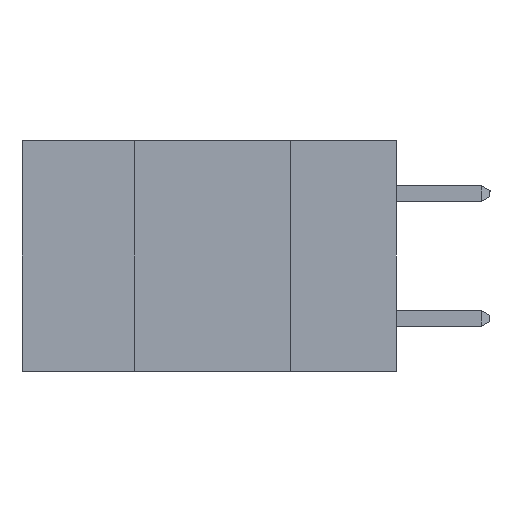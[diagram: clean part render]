
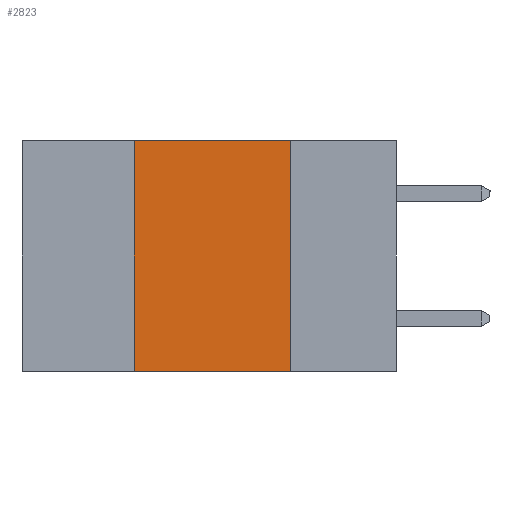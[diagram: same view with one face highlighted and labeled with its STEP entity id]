
A CAD part, left-side view. The second image highlights one B-rep face of the part: STEP entity #2823.
In plain terms, the highlighted planar face has unit normal (-1, 0, 0).
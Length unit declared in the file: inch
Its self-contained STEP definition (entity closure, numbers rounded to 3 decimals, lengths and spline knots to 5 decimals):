
#83 = VERTEX_POINT ( 'NONE', #5161 ) ;
#400 = CARTESIAN_POINT ( 'NONE',  ( 0., 0.42, -0.37 ) ) ;
#405 = DIRECTION ( 'NONE',  ( 0., 0., 1. ) ) ;
#437 = EDGE_CURVE ( 'NONE', #7026, #5167, #7548, .T. ) ;
#523 = CARTESIAN_POINT ( 'NONE',  ( 0., 0.6, 0. ) ) ;
#1561 = CARTESIAN_POINT ( 'NONE',  ( 0., 0.17, 0. ) ) ;
#1673 = CARTESIAN_POINT ( 'NONE',  ( 0., 0.6, 0. ) ) ;
#1726 = DIRECTION ( 'NONE',  ( 0., -1., 0. ) ) ;
#1849 = DIRECTION ( 'NONE',  ( 0., -1., 0. ) ) ;
#1957 = VECTOR ( 'NONE', #1726, 39.37008 ) ;
#2012 = VERTEX_POINT ( 'NONE', #1561 ) ;
#2139 = EDGE_CURVE ( 'NONE', #7026, #83, #5417, .T. ) ;
#2144 = VECTOR ( 'NONE', #5971, 39.37008 ) ;
#2823 = ADVANCED_FACE ( 'NONE', ( #4070 ), #9133, .F. ) ;
#3528 = ORIENTED_EDGE ( 'NONE', *, *, #437, .T. ) ;
#4070 = FACE_OUTER_BOUND ( 'NONE', #4788, .T. ) ;
#4291 = ORIENTED_EDGE ( 'NONE', *, *, #2139, .F. ) ;
#4434 = EDGE_CURVE ( 'NONE', #83, #2012, #7422, .T. ) ;
#4788 = EDGE_LOOP ( 'NONE', ( #5066, #5315, #4291, #3528 ) ) ;
#5066 = ORIENTED_EDGE ( 'NONE', *, *, #7107, .F. ) ;
#5161 = CARTESIAN_POINT ( 'NONE',  ( 0., 0.42, 0. ) ) ;
#5167 = VERTEX_POINT ( 'NONE', #8580 ) ;
#5315 = ORIENTED_EDGE ( 'NONE', *, *, #4434, .F. ) ;
#5417 = LINE ( 'NONE', #6797, #7290 ) ;
#5657 = AXIS2_PLACEMENT_3D ( 'NONE', #523, #8434, #6291 ) ;
#5971 = DIRECTION ( 'NONE',  ( 0., 0., -1. ) ) ;
#6291 = DIRECTION ( 'NONE',  ( 0., 0., -1. ) ) ;
#6797 = CARTESIAN_POINT ( 'NONE',  ( 0., 0.42, -0.37 ) ) ;
#7026 = VERTEX_POINT ( 'NONE', #400 ) ;
#7107 = EDGE_CURVE ( 'NONE', #2012, #5167, #7433, .T. ) ;
#7290 = VECTOR ( 'NONE', #405, 39.37008 ) ;
#7422 = LINE ( 'NONE', #1673, #1957 ) ;
#7433 = LINE ( 'NONE', #7607, #2144 ) ;
#7548 = LINE ( 'NONE', #8185, #8655 ) ;
#7607 = CARTESIAN_POINT ( 'NONE',  ( 0., 0.17, -0.37 ) ) ;
#8185 = CARTESIAN_POINT ( 'NONE',  ( 0., 0.6, -0.37 ) ) ;
#8434 = DIRECTION ( 'NONE',  ( 1., 0., 0. ) ) ;
#8580 = CARTESIAN_POINT ( 'NONE',  ( 0., 0.17, -0.37 ) ) ;
#8655 = VECTOR ( 'NONE', #1849, 39.37008 ) ;
#9133 = PLANE ( 'NONE',  #5657 ) ;
